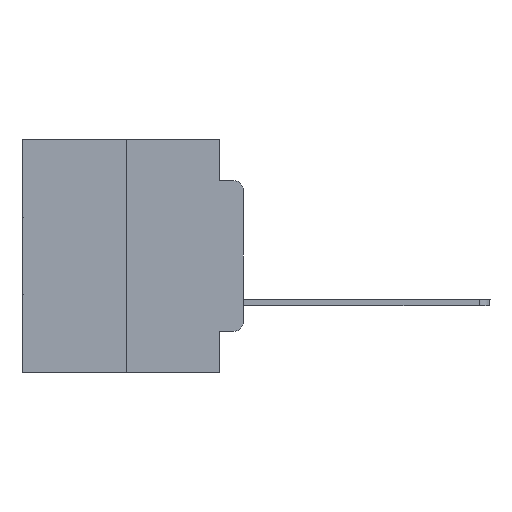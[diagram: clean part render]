
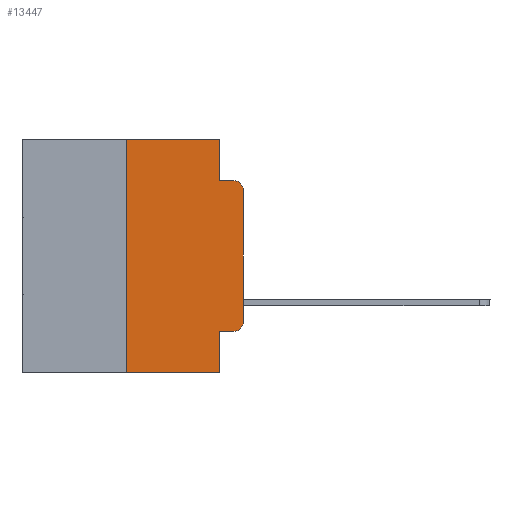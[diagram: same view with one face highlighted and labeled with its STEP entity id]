
A CAD part, left-side view. The second image highlights one B-rep face of the part: STEP entity #13447.
In plain terms, the highlighted planar face has unit normal (-1, 0, 0).
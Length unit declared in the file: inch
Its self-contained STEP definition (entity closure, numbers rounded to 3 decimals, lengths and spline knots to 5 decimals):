
#713 = VERTEX_POINT ( 'NONE', #12519 ) ;
#1001 = CARTESIAN_POINT ( 'NONE',  ( 0., 0.02, -0.1085 ) ) ;
#1469 = DIRECTION ( 'NONE',  ( -1., 0., 0. ) ) ;
#1503 = DIRECTION ( 'NONE',  ( 0., 0., -1. ) ) ;
#2093 = EDGE_CURVE ( 'NONE', #713, #10736, #10635, .T. ) ;
#2182 = VECTOR ( 'NONE', #25552, 39.37008 ) ;
#2669 = CARTESIAN_POINT ( 'NONE',  ( 0., 0.02, -0.3915 ) ) ;
#2788 = VERTEX_POINT ( 'NONE', #27189 ) ;
#2989 = VERTEX_POINT ( 'NONE', #5753 ) ;
#3416 = DIRECTION ( 'NONE',  ( 0., -1., 0. ) ) ;
#3930 = VECTOR ( 'NONE', #5826, 39.37008 ) ;
#4517 = VECTOR ( 'NONE', #26408, 39.37008 ) ;
#4834 = DIRECTION ( 'NONE',  ( 0., 0., -1. ) ) ;
#4928 = ORIENTED_EDGE ( 'NONE', *, *, #10978, .T. ) ;
#5013 = VERTEX_POINT ( 'NONE', #26849 ) ;
#5100 = AXIS2_PLACEMENT_3D ( 'NONE', #2669, #1469, #5666 ) ;
#5389 = ORIENTED_EDGE ( 'NONE', *, *, #2093, .F. ) ;
#5392 = LINE ( 'NONE', #27570, #2182 ) ;
#5500 = CARTESIAN_POINT ( 'NONE',  ( 0., 0., 0. ) ) ;
#5666 = DIRECTION ( 'NONE',  ( 0., 0., -1. ) ) ;
#5753 = CARTESIAN_POINT ( 'NONE',  ( 0., 0.051, 0. ) ) ;
#5826 = DIRECTION ( 'NONE',  ( 0., -1., 0. ) ) ;
#6091 = ORIENTED_EDGE ( 'NONE', *, *, #10548, .F. ) ;
#6132 = EDGE_CURVE ( 'NONE', #21707, #27218, #13256, .T. ) ;
#7041 = EDGE_LOOP ( 'NONE', ( #4928, #10938, #18021, #24219, #24939, #5389, #7196, #6091, #20989, #28230 ) ) ;
#7196 = ORIENTED_EDGE ( 'NONE', *, *, #17479, .T. ) ;
#7441 = CARTESIAN_POINT ( 'NONE',  ( 0., 0.051, -0.5 ) ) ;
#7775 = CARTESIAN_POINT ( 'NONE',  ( 0., 0.473, -0.5 ) ) ;
#7823 = DIRECTION ( 'NONE',  ( 0., 0., -1. ) ) ;
#9054 = CARTESIAN_POINT ( 'NONE',  ( 0., 0.473, 0. ) ) ;
#9102 = EDGE_CURVE ( 'NONE', #2989, #21707, #14668, .T. ) ;
#10203 = VECTOR ( 'NONE', #24558, 39.37008 ) ;
#10548 = EDGE_CURVE ( 'NONE', #16266, #11879, #5392, .T. ) ;
#10635 = LINE ( 'NONE', #12931, #4517 ) ;
#10736 = VERTEX_POINT ( 'NONE', #17269 ) ;
#10938 = ORIENTED_EDGE ( 'NONE', *, *, #22816, .T. ) ;
#10978 = EDGE_CURVE ( 'NONE', #2788, #5013, #11867, .T. ) ;
#11867 = LINE ( 'NONE', #5500, #15615 ) ;
#11879 = VERTEX_POINT ( 'NONE', #7441 ) ;
#12502 = AXIS2_PLACEMENT_3D ( 'NONE', #1001, #16784, #7823 ) ;
#12519 = CARTESIAN_POINT ( 'NONE',  ( 0., 0.25, -0.5 ) ) ;
#12931 = CARTESIAN_POINT ( 'NONE',  ( 0., 0.25, 0. ) ) ;
#13256 = LINE ( 'NONE', #22105, #25019 ) ;
#13447 = ADVANCED_FACE ( 'NONE', ( #15546 ), #24406, .F. ) ;
#14668 = LINE ( 'NONE', #21067, #18440 ) ;
#14826 = EDGE_CURVE ( 'NONE', #10736, #2989, #15409, .T. ) ;
#15409 = LINE ( 'NONE', #26570, #10203 ) ;
#15546 = FACE_OUTER_BOUND ( 'NONE', #7041, .T. ) ;
#15615 = VECTOR ( 'NONE', #20854, 39.37008 ) ;
#15679 = DIRECTION ( 'NONE',  ( 1., 0., 0. ) ) ;
#16266 = VERTEX_POINT ( 'NONE', #26255 ) ;
#16784 = DIRECTION ( 'NONE',  ( -1., 0., 0. ) ) ;
#17269 = CARTESIAN_POINT ( 'NONE',  ( 0., 0.25, 0. ) ) ;
#17479 = EDGE_CURVE ( 'NONE', #713, #11879, #25316, .T. ) ;
#17760 = DIRECTION ( 'NONE',  ( 0., -1., 0. ) ) ;
#18021 = ORIENTED_EDGE ( 'NONE', *, *, #6132, .F. ) ;
#18440 = VECTOR ( 'NONE', #1503, 39.37008 ) ;
#18952 = AXIS2_PLACEMENT_3D ( 'NONE', #9054, #15679, #4834 ) ;
#20428 = CARTESIAN_POINT ( 'NONE',  ( 0., 0.02, -0.0885 ) ) ;
#20783 = EDGE_CURVE ( 'NONE', #16266, #21577, #25697, .T. ) ;
#20854 = DIRECTION ( 'NONE',  ( 0., 0., 1. ) ) ;
#20989 = ORIENTED_EDGE ( 'NONE', *, *, #20783, .T. ) ;
#21067 = CARTESIAN_POINT ( 'NONE',  ( 0., 0.051, 0. ) ) ;
#21175 = CARTESIAN_POINT ( 'NONE',  ( 0., 0.051, -0.4115 ) ) ;
#21577 = VERTEX_POINT ( 'NONE', #23012 ) ;
#21707 = VERTEX_POINT ( 'NONE', #25921 ) ;
#21762 = CIRCLE ( 'NONE', #5100, 0.02 ) ;
#22105 = CARTESIAN_POINT ( 'NONE',  ( 0., 0.051, -0.0885 ) ) ;
#22409 = EDGE_CURVE ( 'NONE', #21577, #2788, #21762, .T. ) ;
#22816 = EDGE_CURVE ( 'NONE', #5013, #27218, #26789, .T. ) ;
#23012 = CARTESIAN_POINT ( 'NONE',  ( 0., 0.02, -0.4115 ) ) ;
#24219 = ORIENTED_EDGE ( 'NONE', *, *, #9102, .F. ) ;
#24406 = PLANE ( 'NONE',  #18952 ) ;
#24558 = DIRECTION ( 'NONE',  ( 0., -1., 0. ) ) ;
#24939 = ORIENTED_EDGE ( 'NONE', *, *, #14826, .F. ) ;
#25019 = VECTOR ( 'NONE', #17760, 39.37008 ) ;
#25131 = VECTOR ( 'NONE', #3416, 39.37008 ) ;
#25316 = LINE ( 'NONE', #7775, #25131 ) ;
#25552 = DIRECTION ( 'NONE',  ( 0., 0., -1. ) ) ;
#25697 = LINE ( 'NONE', #21175, #3930 ) ;
#25921 = CARTESIAN_POINT ( 'NONE',  ( 0., 0.051, -0.0885 ) ) ;
#26255 = CARTESIAN_POINT ( 'NONE',  ( 0., 0.051, -0.4115 ) ) ;
#26408 = DIRECTION ( 'NONE',  ( 0., 0., 1. ) ) ;
#26570 = CARTESIAN_POINT ( 'NONE',  ( 0., 0.473, 0. ) ) ;
#26789 = CIRCLE ( 'NONE', #12502, 0.02 ) ;
#26849 = CARTESIAN_POINT ( 'NONE',  ( 0., 0., -0.1085 ) ) ;
#27189 = CARTESIAN_POINT ( 'NONE',  ( 0., 0., -0.3915 ) ) ;
#27218 = VERTEX_POINT ( 'NONE', #20428 ) ;
#27570 = CARTESIAN_POINT ( 'NONE',  ( 0., 0.051, 0. ) ) ;
#28230 = ORIENTED_EDGE ( 'NONE', *, *, #22409, .T. ) ;
